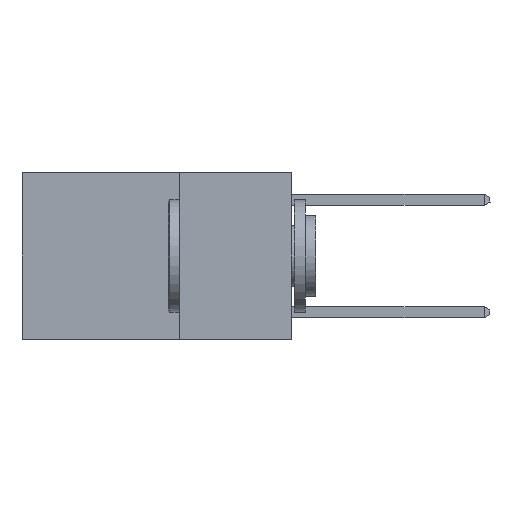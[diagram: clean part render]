
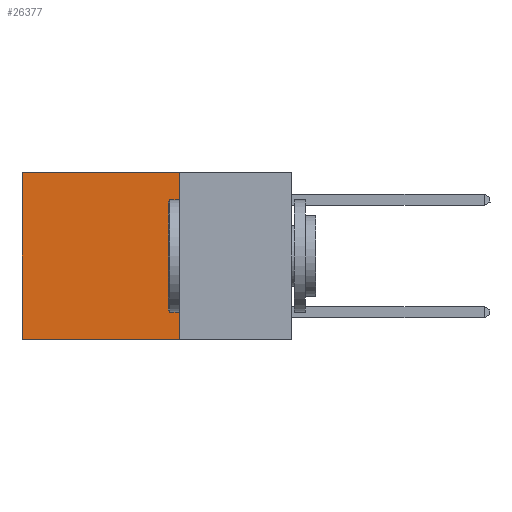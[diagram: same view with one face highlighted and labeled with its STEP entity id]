
A CAD part, left-side view. The second image highlights one B-rep face of the part: STEP entity #26377.
In plain terms, the highlighted planar face has unit normal (-1, 0, 0).
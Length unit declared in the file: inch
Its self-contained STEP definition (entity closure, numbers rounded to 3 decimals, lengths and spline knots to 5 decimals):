
#2382 = FACE_OUTER_BOUND ( 'NONE', #15340, .T. ) ;
#3735 = VERTEX_POINT ( 'NONE', #24258 ) ;
#3745 = DIRECTION ( 'NONE',  ( 0., 0., -1. ) ) ;
#3856 = CARTESIAN_POINT ( 'NONE',  ( 0.2625, 0.25, 0. ) ) ;
#4476 = EDGE_CURVE ( 'NONE', #24722, #3735, #24444, .T. ) ;
#5442 = LINE ( 'NONE', #29755, #9582 ) ;
#6100 = EDGE_CURVE ( 'NONE', #8945, #22703, #31184, .T. ) ;
#6973 = DIRECTION ( 'NONE',  ( 0., 1., 0. ) ) ;
#8945 = VERTEX_POINT ( 'NONE', #22865 ) ;
#9582 = VECTOR ( 'NONE', #12988, 39.37008 ) ;
#9881 = CARTESIAN_POINT ( 'NONE',  ( 0.2625, 0.25, 0. ) ) ;
#9890 = AXIS2_PLACEMENT_3D ( 'NONE', #3856, #25603, #3745 ) ;
#10331 = EDGE_CURVE ( 'NONE', #3735, #22703, #5442, .T. ) ;
#12463 = CARTESIAN_POINT ( 'NONE',  ( 0.2625, 0.6, -0.37 ) ) ;
#12988 = DIRECTION ( 'NONE',  ( 0., 0., -1. ) ) ;
#13691 = VECTOR ( 'NONE', #18588, 39.37008 ) ;
#14218 = CARTESIAN_POINT ( 'NONE',  ( 0.2625, 0.25, -0.37 ) ) ;
#15340 = EDGE_LOOP ( 'NONE', ( #16246, #19618, #22643, #17837 ) ) ;
#16246 = ORIENTED_EDGE ( 'NONE', *, *, #10331, .T. ) ;
#17808 = DIRECTION ( 'NONE',  ( 0., 1., 0. ) ) ;
#17837 = ORIENTED_EDGE ( 'NONE', *, *, #4476, .T. ) ;
#18227 = EDGE_CURVE ( 'NONE', #24722, #8945, #26529, .T. ) ;
#18588 = DIRECTION ( 'NONE',  ( 0., 0., -1. ) ) ;
#19043 = PLANE ( 'NONE',  #9890 ) ;
#19618 = ORIENTED_EDGE ( 'NONE', *, *, #6100, .F. ) ;
#22643 = ORIENTED_EDGE ( 'NONE', *, *, #18227, .F. ) ;
#22703 = VERTEX_POINT ( 'NONE', #12463 ) ;
#22865 = CARTESIAN_POINT ( 'NONE',  ( 0.2625, 0.25, -0.37 ) ) ;
#24009 = VECTOR ( 'NONE', #6973, 39.37008 ) ;
#24258 = CARTESIAN_POINT ( 'NONE',  ( 0.2625, 0.6, 0. ) ) ;
#24444 = LINE ( 'NONE', #27412, #27472 ) ;
#24722 = VERTEX_POINT ( 'NONE', #9881 ) ;
#25603 = DIRECTION ( 'NONE',  ( 1., 0., 0. ) ) ;
#26377 = ADVANCED_FACE ( 'NONE', ( #2382 ), #19043, .F. ) ;
#26529 = LINE ( 'NONE', #30518, #13691 ) ;
#27412 = CARTESIAN_POINT ( 'NONE',  ( 0.2625, 0.25, 0. ) ) ;
#27472 = VECTOR ( 'NONE', #17808, 39.37008 ) ;
#29755 = CARTESIAN_POINT ( 'NONE',  ( 0.2625, 0.6, 0. ) ) ;
#30518 = CARTESIAN_POINT ( 'NONE',  ( 0.2625, 0.25, 0. ) ) ;
#31184 = LINE ( 'NONE', #14218, #24009 ) ;
